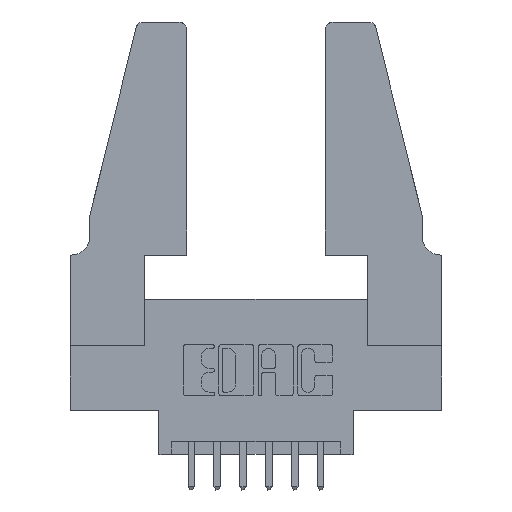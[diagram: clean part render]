
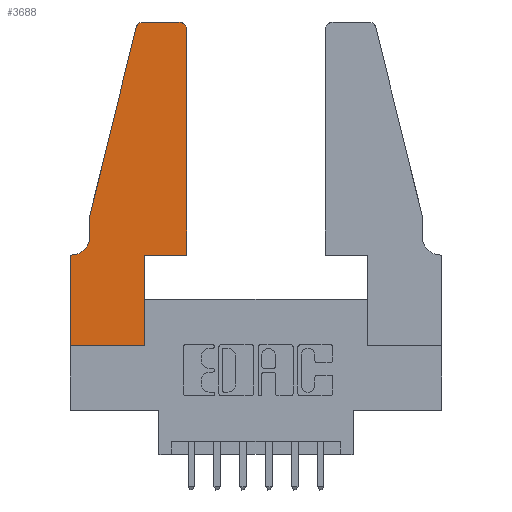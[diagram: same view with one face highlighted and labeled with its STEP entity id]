
A CAD part, top view. The second image highlights one B-rep face of the part: STEP entity #3688.
In plain terms, the highlighted planar face has unit normal (0, 0, 1).
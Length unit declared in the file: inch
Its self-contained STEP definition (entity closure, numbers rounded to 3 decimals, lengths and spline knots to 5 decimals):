
#149 = DIRECTION ( 'NONE',  ( 0., 1., 0. ) ) ;
#269 = DIRECTION ( 'NONE',  ( -0.239, -0.971, 0. ) ) ;
#276 = EDGE_CURVE ( 'NONE', #8201, #6996, #2641, .T. ) ;
#466 = VECTOR ( 'NONE', #269, 39.37008 ) ;
#617 = LINE ( 'NONE', #8146, #7655 ) ;
#653 = ORIENTED_EDGE ( 'NONE', *, *, #2258, .T. ) ;
#736 = EDGE_CURVE ( 'NONE', #11704, #6975, #2495, .T. ) ;
#1009 = PLANE ( 'NONE',  #3156 ) ;
#1050 = ORIENTED_EDGE ( 'NONE', *, *, #11338, .T. ) ;
#1060 = CARTESIAN_POINT ( 'NONE',  ( 0.4505, 0.35, 0.37 ) ) ;
#1096 = DIRECTION ( 'NONE',  ( 1., 0., 0. ) ) ;
#1122 = EDGE_CURVE ( 'NONE', #11285, #2122, #3655, .T. ) ;
#1168 = VECTOR ( 'NONE', #11367, 39.37008 ) ;
#1201 = CARTESIAN_POINT ( 'NONE',  ( 0.0755, 0.5, 0.37 ) ) ;
#1413 = VECTOR ( 'NONE', #2123, 39.37008 ) ;
#1657 = LINE ( 'NONE', #1060, #11434 ) ;
#1920 = DIRECTION ( 'NONE',  ( 1., 0., 0. ) ) ;
#2122 = VERTEX_POINT ( 'NONE', #6558 ) ;
#2123 = DIRECTION ( 'NONE',  ( 0., -1., 0. ) ) ;
#2258 = EDGE_CURVE ( 'NONE', #4984, #11285, #8367, .T. ) ;
#2356 = AXIS2_PLACEMENT_3D ( 'NONE', #6829, #6777, #7353 ) ;
#2495 = CIRCLE ( 'NONE', #2356, 0.07 ) ;
#2512 = ORIENTED_EDGE ( 'NONE', *, *, #736, .T. ) ;
#2641 = CIRCLE ( 'NONE', #7115, 0.03 ) ;
#2897 = DIRECTION ( 'NONE',  ( 0., 0., 1. ) ) ;
#3156 = AXIS2_PLACEMENT_3D ( 'NONE', #4679, #7443, #1920 ) ;
#3247 = VERTEX_POINT ( 'NONE', #10421 ) ;
#3272 = CARTESIAN_POINT ( 'NONE',  ( 0.0755, 0.5, 0.37 ) ) ;
#3483 = VECTOR ( 'NONE', #8079, 39.37008 ) ;
#3655 = LINE ( 'NONE', #7691, #3953 ) ;
#3688 = ADVANCED_FACE ( 'NONE', ( #7746 ), #1009, .T. ) ;
#3766 = ORIENTED_EDGE ( 'NONE', *, *, #8442, .T. ) ;
#3814 = CARTESIAN_POINT ( 'NONE',  ( 0.2865, 0.35, 0.37 ) ) ;
#3827 = EDGE_CURVE ( 'NONE', #9209, #11704, #8770, .T. ) ;
#3953 = VECTOR ( 'NONE', #7639, 39.37008 ) ;
#3985 = ORIENTED_EDGE ( 'NONE', *, *, #11700, .T. ) ;
#4003 = ORIENTED_EDGE ( 'NONE', *, *, #276, .T. ) ;
#4057 = CARTESIAN_POINT ( 'NONE',  ( 0., 0., 0.37 ) ) ;
#4403 = CARTESIAN_POINT ( 'NONE',  ( 0.284, 1.25, 0.37 ) ) ;
#4413 = CARTESIAN_POINT ( 'NONE',  ( 0.2865, 0.35, 0.37 ) ) ;
#4679 = CARTESIAN_POINT ( 'NONE',  ( 0., 0.35, 0.37 ) ) ;
#4956 = CARTESIAN_POINT ( 'NONE',  ( 0.0755, 0.42, 0.37 ) ) ;
#4984 = VERTEX_POINT ( 'NONE', #7455 ) ;
#5012 = EDGE_CURVE ( 'NONE', #2122, #8201, #1657, .T. ) ;
#5226 = ORIENTED_EDGE ( 'NONE', *, *, #7228, .T. ) ;
#5568 = ORIENTED_EDGE ( 'NONE', *, *, #1122, .T. ) ;
#5793 = CARTESIAN_POINT ( 'NONE',  ( 0., 0., 0.37 ) ) ;
#5871 = LINE ( 'NONE', #6595, #10471 ) ;
#5934 = VERTEX_POINT ( 'NONE', #5990 ) ;
#5954 = CIRCLE ( 'NONE', #6842, 0.03 ) ;
#5990 = CARTESIAN_POINT ( 'NONE',  ( 0., 0.35, 0.37 ) ) ;
#6213 = VECTOR ( 'NONE', #7897, 39.37008 ) ;
#6283 = DIRECTION ( 'NONE',  ( -1., 0., 0. ) ) ;
#6338 = EDGE_CURVE ( 'NONE', #8730, #3247, #5954, .T. ) ;
#6558 = CARTESIAN_POINT ( 'NONE',  ( 0.4505, 0.35, 0.37 ) ) ;
#6595 = CARTESIAN_POINT ( 'NONE',  ( 0., 0., 0.37 ) ) ;
#6597 = CARTESIAN_POINT ( 'NONE',  ( 0.4205, 1.25, 0.37 ) ) ;
#6667 = CARTESIAN_POINT ( 'NONE',  ( 0.0755, 0.5, 0.37 ) ) ;
#6777 = DIRECTION ( 'NONE',  ( 0., 0., -1. ) ) ;
#6829 = CARTESIAN_POINT ( 'NONE',  ( 0.0055, 0.42, 0.37 ) ) ;
#6842 = AXIS2_PLACEMENT_3D ( 'NONE', #8406, #2897, #9325 ) ;
#6950 = CARTESIAN_POINT ( 'NONE',  ( 0.2605, 1.25, 0.37 ) ) ;
#6975 = VERTEX_POINT ( 'NONE', #11177 ) ;
#6996 = VERTEX_POINT ( 'NONE', #6597 ) ;
#7115 = AXIS2_PLACEMENT_3D ( 'NONE', #11132, #10329, #10373 ) ;
#7228 = EDGE_CURVE ( 'NONE', #6996, #8730, #8960, .T. ) ;
#7353 = DIRECTION ( 'NONE',  ( -1., 0., 0. ) ) ;
#7443 = DIRECTION ( 'NONE',  ( 0., 0., 1. ) ) ;
#7455 = CARTESIAN_POINT ( 'NONE',  ( 0.2865, 0., 0.37 ) ) ;
#7639 = DIRECTION ( 'NONE',  ( 1., 0., 0. ) ) ;
#7655 = VECTOR ( 'NONE', #6283, 39.37008 ) ;
#7691 = CARTESIAN_POINT ( 'NONE',  ( 0.4505, 0.35, 0.37 ) ) ;
#7701 = ORIENTED_EDGE ( 'NONE', *, *, #3827, .T. ) ;
#7746 = FACE_OUTER_BOUND ( 'NONE', #10596, .T. ) ;
#7785 = ORIENTED_EDGE ( 'NONE', *, *, #6338, .T. ) ;
#7897 = DIRECTION ( 'NONE',  ( -1., 0., 0. ) ) ;
#8079 = DIRECTION ( 'NONE',  ( 0., 1., 0. ) ) ;
#8146 = CARTESIAN_POINT ( 'NONE',  ( 0.0755, 0.35, 0.37 ) ) ;
#8201 = VERTEX_POINT ( 'NONE', #11819 ) ;
#8367 = LINE ( 'NONE', #3814, #3483 ) ;
#8406 = CARTESIAN_POINT ( 'NONE',  ( 0.284, 1.22, 0.37 ) ) ;
#8442 = EDGE_CURVE ( 'NONE', #3247, #9209, #10802, .T. ) ;
#8730 = VERTEX_POINT ( 'NONE', #4403 ) ;
#8770 = LINE ( 'NONE', #1201, #1413 ) ;
#8817 = LINE ( 'NONE', #4057, #1168 ) ;
#8960 = LINE ( 'NONE', #6950, #6213 ) ;
#9031 = ORIENTED_EDGE ( 'NONE', *, *, #10252, .T. ) ;
#9209 = VERTEX_POINT ( 'NONE', #3272 ) ;
#9325 = DIRECTION ( 'NONE',  ( 1., 0., 0. ) ) ;
#10252 = EDGE_CURVE ( 'NONE', #11643, #4984, #5871, .T. ) ;
#10329 = DIRECTION ( 'NONE',  ( 0., 0., 1. ) ) ;
#10373 = DIRECTION ( 'NONE',  ( 1., 0., 0. ) ) ;
#10421 = CARTESIAN_POINT ( 'NONE',  ( 0.25487, 1.22718, 0.37 ) ) ;
#10471 = VECTOR ( 'NONE', #1096, 39.37008 ) ;
#10596 = EDGE_LOOP ( 'NONE', ( #5226, #7785, #3766, #7701, #2512, #1050, #3985, #9031, #653, #5568, #11883, #4003 ) ) ;
#10802 = LINE ( 'NONE', #6667, #466 ) ;
#11132 = CARTESIAN_POINT ( 'NONE',  ( 0.4205, 1.22, 0.37 ) ) ;
#11177 = CARTESIAN_POINT ( 'NONE',  ( 0.0055, 0.35, 0.37 ) ) ;
#11285 = VERTEX_POINT ( 'NONE', #4413 ) ;
#11338 = EDGE_CURVE ( 'NONE', #6975, #5934, #617, .T. ) ;
#11367 = DIRECTION ( 'NONE',  ( 0., -1., 0. ) ) ;
#11434 = VECTOR ( 'NONE', #149, 39.37008 ) ;
#11643 = VERTEX_POINT ( 'NONE', #5793 ) ;
#11700 = EDGE_CURVE ( 'NONE', #5934, #11643, #8817, .T. ) ;
#11704 = VERTEX_POINT ( 'NONE', #4956 ) ;
#11819 = CARTESIAN_POINT ( 'NONE',  ( 0.4505, 1.22, 0.37 ) ) ;
#11883 = ORIENTED_EDGE ( 'NONE', *, *, #5012, .T. ) ;
